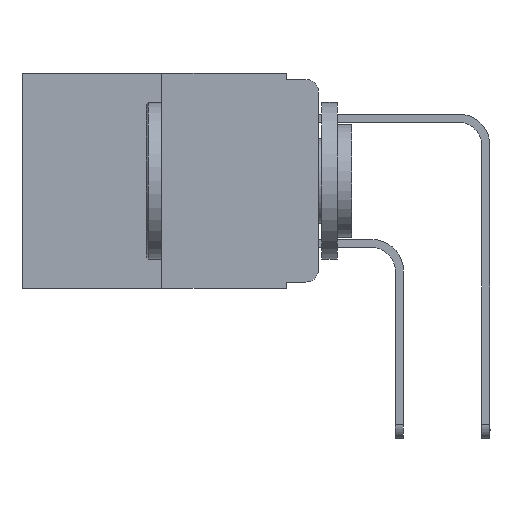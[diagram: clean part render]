
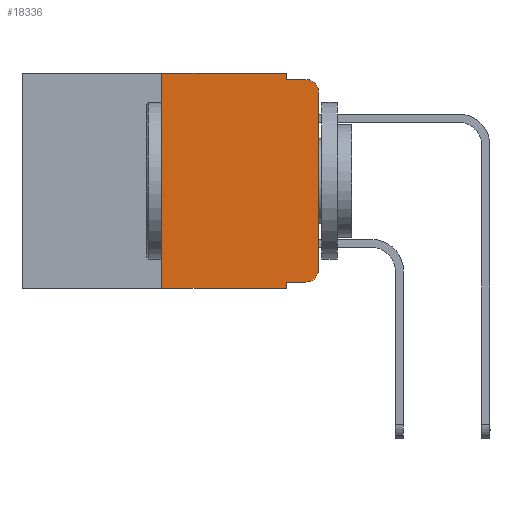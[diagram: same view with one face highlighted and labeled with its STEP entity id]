
A CAD part, left-side view. The second image highlights one B-rep face of the part: STEP entity #18336.
In plain terms, the highlighted planar face has unit normal (-1, 0, 0).
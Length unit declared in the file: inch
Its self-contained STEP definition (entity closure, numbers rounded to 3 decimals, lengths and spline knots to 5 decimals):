
#93 = EDGE_CURVE ( 'NONE', #8976, #23379, #22542, .T. ) ;
#676 = VECTOR ( 'NONE', #19040, 39.37008 ) ;
#1450 = ORIENTED_EDGE ( 'NONE', *, *, #17959, .T. ) ;
#1635 = DIRECTION ( 'NONE',  ( 0., 0., -1. ) ) ;
#1651 = VECTOR ( 'NONE', #6356, 39.37008 ) ;
#2452 = ORIENTED_EDGE ( 'NONE', *, *, #21867, .F. ) ;
#2689 = ORIENTED_EDGE ( 'NONE', *, *, #6885, .F. ) ;
#3075 = CARTESIAN_POINT ( 'NONE',  ( 0., 0.02, -0.01 ) ) ;
#3231 = DIRECTION ( 'NONE',  ( 0., 0., -1. ) ) ;
#4175 = EDGE_CURVE ( 'NONE', #14649, #24428, #14484, .T. ) ;
#4185 = CARTESIAN_POINT ( 'NONE',  ( 0., 0.25, 0. ) ) ;
#4343 = EDGE_CURVE ( 'NONE', #24428, #23379, #6767, .T. ) ;
#4383 = ORIENTED_EDGE ( 'NONE', *, *, #11447, .T. ) ;
#4395 = VECTOR ( 'NONE', #17274, 39.37008 ) ;
#4450 = CARTESIAN_POINT ( 'NONE',  ( 0., 0.051, -0.333 ) ) ;
#4744 = DIRECTION ( 'NONE',  ( -1., 0., 0. ) ) ;
#4948 = VERTEX_POINT ( 'NONE', #19601 ) ;
#5476 = CARTESIAN_POINT ( 'NONE',  ( 0., 0.051, 0. ) ) ;
#5828 = VECTOR ( 'NONE', #13813, 39.37008 ) ;
#6064 = ORIENTED_EDGE ( 'NONE', *, *, #12683, .T. ) ;
#6191 = EDGE_CURVE ( 'NONE', #17276, #20283, #23303, .T. ) ;
#6356 = DIRECTION ( 'NONE',  ( 0., -1., 0. ) ) ;
#6416 = DIRECTION ( 'NONE',  ( 0., -1., 0. ) ) ;
#6641 = CARTESIAN_POINT ( 'NONE',  ( 0., 0.25, -0.343 ) ) ;
#6767 = CIRCLE ( 'NONE', #12379, 0.02 ) ;
#6885 = EDGE_CURVE ( 'NONE', #12959, #19919, #14069, .T. ) ;
#8179 = ORIENTED_EDGE ( 'NONE', *, *, #4343, .T. ) ;
#8576 = CARTESIAN_POINT ( 'NONE',  ( 0., 0.473, 0. ) ) ;
#8976 = VERTEX_POINT ( 'NONE', #22535 ) ;
#9038 = VECTOR ( 'NONE', #21314, 39.37008 ) ;
#9558 = EDGE_LOOP ( 'NONE', ( #18569, #8179, #18866, #12633, #2452, #23555, #1450, #2689, #6064, #4383 ) ) ;
#10051 = CARTESIAN_POINT ( 'NONE',  ( 0., 0.25, 0. ) ) ;
#10641 = DIRECTION ( 'NONE',  ( 0., 0., -1. ) ) ;
#11398 = EDGE_CURVE ( 'NONE', #13582, #8976, #17469, .T. ) ;
#11447 = EDGE_CURVE ( 'NONE', #4948, #14649, #24529, .T. ) ;
#11906 = CARTESIAN_POINT ( 'NONE',  ( 0., 0., -0.03 ) ) ;
#12379 = AXIS2_PLACEMENT_3D ( 'NONE', #21559, #4744, #18000 ) ;
#12382 = VECTOR ( 'NONE', #1635, 39.37008 ) ;
#12633 = ORIENTED_EDGE ( 'NONE', *, *, #11398, .F. ) ;
#12683 = EDGE_CURVE ( 'NONE', #12959, #4948, #18844, .T. ) ;
#12959 = VERTEX_POINT ( 'NONE', #20168 ) ;
#13582 = VERTEX_POINT ( 'NONE', #5476 ) ;
#13615 = CARTESIAN_POINT ( 'NONE',  ( 0., 0., 0. ) ) ;
#13813 = DIRECTION ( 'NONE',  ( 0., -1., 0. ) ) ;
#14069 = LINE ( 'NONE', #23358, #9038 ) ;
#14359 = DIRECTION ( 'NONE',  ( 1., 0., 0. ) ) ;
#14362 = CARTESIAN_POINT ( 'NONE',  ( 0., 0.473, -0.343 ) ) ;
#14484 = LINE ( 'NONE', #13615, #4395 ) ;
#14649 = VERTEX_POINT ( 'NONE', #22100 ) ;
#16402 = LINE ( 'NONE', #14362, #676 ) ;
#16735 = CARTESIAN_POINT ( 'NONE',  ( 0., 0.051, 0. ) ) ;
#16980 = FACE_OUTER_BOUND ( 'NONE', #9558, .T. ) ;
#17274 = DIRECTION ( 'NONE',  ( 0., 0., 1. ) ) ;
#17276 = VERTEX_POINT ( 'NONE', #6641 ) ;
#17469 = LINE ( 'NONE', #16735, #12382 ) ;
#17862 = CARTESIAN_POINT ( 'NONE',  ( 0., 0.051, -0.01 ) ) ;
#17959 = EDGE_CURVE ( 'NONE', #17276, #19919, #16402, .T. ) ;
#18000 = DIRECTION ( 'NONE',  ( 0., 0., -1. ) ) ;
#18122 = CARTESIAN_POINT ( 'NONE',  ( 0., 0.051, -0.343 ) ) ;
#18243 = DIRECTION ( 'NONE',  ( -1., 0., 0. ) ) ;
#18336 = ADVANCED_FACE ( 'NONE', ( #16980 ), #19957, .F. ) ;
#18435 = AXIS2_PLACEMENT_3D ( 'NONE', #8576, #14359, #10641 ) ;
#18526 = AXIS2_PLACEMENT_3D ( 'NONE', #24107, #18243, #3231 ) ;
#18569 = ORIENTED_EDGE ( 'NONE', *, *, #4175, .T. ) ;
#18844 = LINE ( 'NONE', #4450, #1651 ) ;
#18866 = ORIENTED_EDGE ( 'NONE', *, *, #93, .F. ) ;
#19040 = DIRECTION ( 'NONE',  ( 0., -1., 0. ) ) ;
#19593 = DIRECTION ( 'NONE',  ( 0., 0., 1. ) ) ;
#19601 = CARTESIAN_POINT ( 'NONE',  ( 0., 0.02, -0.333 ) ) ;
#19919 = VERTEX_POINT ( 'NONE', #18122 ) ;
#19957 = PLANE ( 'NONE',  #18435 ) ;
#20168 = CARTESIAN_POINT ( 'NONE',  ( 0., 0.051, -0.333 ) ) ;
#20283 = VERTEX_POINT ( 'NONE', #4185 ) ;
#21072 = CARTESIAN_POINT ( 'NONE',  ( 0., 0.473, 0. ) ) ;
#21314 = DIRECTION ( 'NONE',  ( 0., 0., -1. ) ) ;
#21559 = CARTESIAN_POINT ( 'NONE',  ( 0., 0.02, -0.03 ) ) ;
#21826 = LINE ( 'NONE', #21072, #5828 ) ;
#21867 = EDGE_CURVE ( 'NONE', #20283, #13582, #21826, .T. ) ;
#22100 = CARTESIAN_POINT ( 'NONE',  ( 0., 0., -0.313 ) ) ;
#22535 = CARTESIAN_POINT ( 'NONE',  ( 0., 0.051, -0.01 ) ) ;
#22542 = LINE ( 'NONE', #17862, #22829 ) ;
#22734 = VECTOR ( 'NONE', #19593, 39.37008 ) ;
#22829 = VECTOR ( 'NONE', #6416, 39.37008 ) ;
#23303 = LINE ( 'NONE', #10051, #22734 ) ;
#23358 = CARTESIAN_POINT ( 'NONE',  ( 0., 0.051, 0. ) ) ;
#23379 = VERTEX_POINT ( 'NONE', #3075 ) ;
#23555 = ORIENTED_EDGE ( 'NONE', *, *, #6191, .F. ) ;
#24107 = CARTESIAN_POINT ( 'NONE',  ( 0., 0.02, -0.313 ) ) ;
#24428 = VERTEX_POINT ( 'NONE', #11906 ) ;
#24529 = CIRCLE ( 'NONE', #18526, 0.02 ) ;
